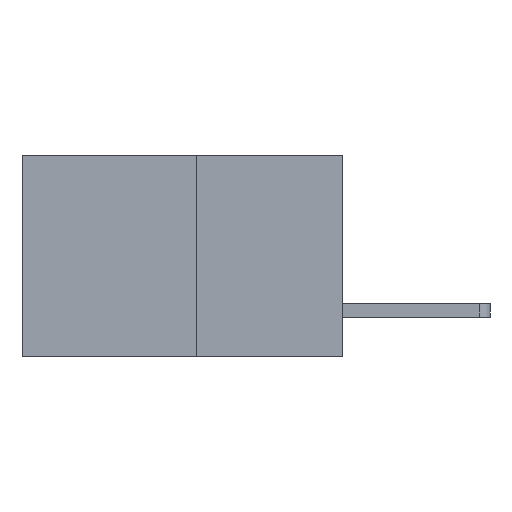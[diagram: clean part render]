
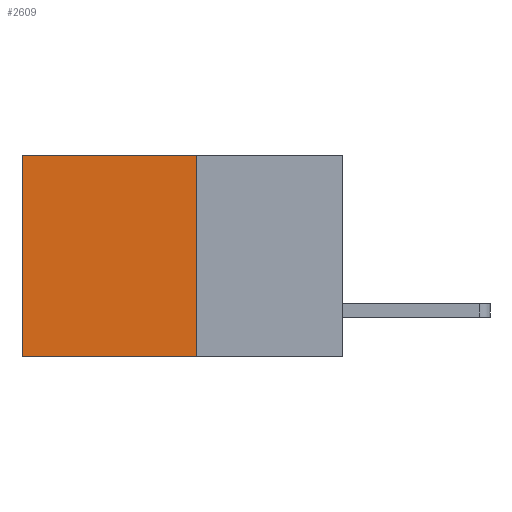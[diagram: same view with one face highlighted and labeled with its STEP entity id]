
A CAD part, left-side view. The second image highlights one B-rep face of the part: STEP entity #2609.
In plain terms, the highlighted planar face has unit normal (-1, 0, 0).
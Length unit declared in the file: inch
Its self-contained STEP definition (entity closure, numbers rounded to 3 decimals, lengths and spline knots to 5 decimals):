
#70 = ORIENTED_EDGE ( 'NONE', *, *, #362, .F. ) ;
#83 = EDGE_LOOP ( 'NONE', ( #7816, #70, #496, #505 ) ) ;
#362 = EDGE_CURVE ( 'NONE', #6212, #597, #6455, .T. ) ;
#496 = ORIENTED_EDGE ( 'NONE', *, *, #5543, .F. ) ;
#505 = ORIENTED_EDGE ( 'NONE', *, *, #3483, .T. ) ;
#597 = VERTEX_POINT ( 'NONE', #3070 ) ;
#833 = CARTESIAN_POINT ( 'NONE',  ( 0.277, 0.59, -0.37 ) ) ;
#1271 = VECTOR ( 'NONE', #3009, 39.37008 ) ;
#1651 = DIRECTION ( 'NONE',  ( 0., 0., -1. ) ) ;
#1678 = CARTESIAN_POINT ( 'NONE',  ( 0.277, 0.27, 0. ) ) ;
#1778 = LINE ( 'NONE', #1678, #3730 ) ;
#2065 = VERTEX_POINT ( 'NONE', #5396 ) ;
#2098 = PLANE ( 'NONE',  #5039 ) ;
#2360 = VERTEX_POINT ( 'NONE', #2703 ) ;
#2609 = ADVANCED_FACE ( 'NONE', ( #6255 ), #2098, .F. ) ;
#2703 = CARTESIAN_POINT ( 'NONE',  ( 0.277, 0.59, 0. ) ) ;
#3009 = DIRECTION ( 'NONE',  ( 0., 0., -1. ) ) ;
#3070 = CARTESIAN_POINT ( 'NONE',  ( 0.277, 0.59, -0.37 ) ) ;
#3125 = CARTESIAN_POINT ( 'NONE',  ( 0.277, 0.27, -0.37 ) ) ;
#3306 = LINE ( 'NONE', #833, #6421 ) ;
#3483 = EDGE_CURVE ( 'NONE', #2065, #2360, #1778, .T. ) ;
#3622 = CARTESIAN_POINT ( 'NONE',  ( 0.277, 0.27, -0.37 ) ) ;
#3730 = VECTOR ( 'NONE', #6057, 39.37008 ) ;
#3990 = DIRECTION ( 'NONE',  ( 1., 0., 0. ) ) ;
#4338 = CARTESIAN_POINT ( 'NONE',  ( 0.277, 0.27, -0.37 ) ) ;
#4826 = VECTOR ( 'NONE', #5253, 39.37008 ) ;
#4872 = EDGE_CURVE ( 'NONE', #2360, #597, #3306, .T. ) ;
#5039 = AXIS2_PLACEMENT_3D ( 'NONE', #3622, #3990, #7567 ) ;
#5101 = CARTESIAN_POINT ( 'NONE',  ( 0.277, 0.27, -0.37 ) ) ;
#5253 = DIRECTION ( 'NONE',  ( 0., 1., 0. ) ) ;
#5396 = CARTESIAN_POINT ( 'NONE',  ( 0.277, 0.27, 0. ) ) ;
#5543 = EDGE_CURVE ( 'NONE', #2065, #6212, #6513, .T. ) ;
#6057 = DIRECTION ( 'NONE',  ( 0., 1., 0. ) ) ;
#6212 = VERTEX_POINT ( 'NONE', #4338 ) ;
#6255 = FACE_OUTER_BOUND ( 'NONE', #83, .T. ) ;
#6421 = VECTOR ( 'NONE', #1651, 39.37008 ) ;
#6455 = LINE ( 'NONE', #5101, #4826 ) ;
#6513 = LINE ( 'NONE', #3125, #1271 ) ;
#7567 = DIRECTION ( 'NONE',  ( 0., 0., -1. ) ) ;
#7816 = ORIENTED_EDGE ( 'NONE', *, *, #4872, .T. ) ;
